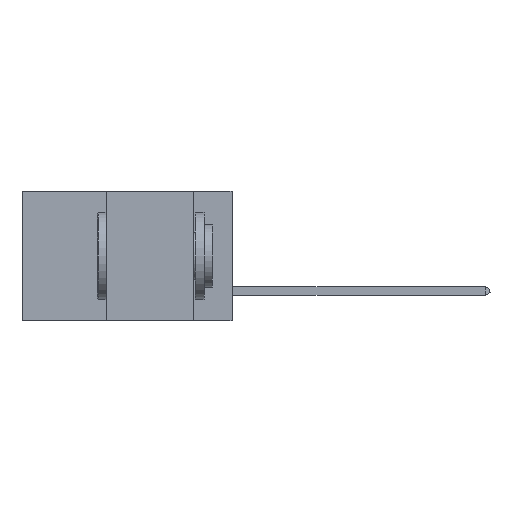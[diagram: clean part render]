
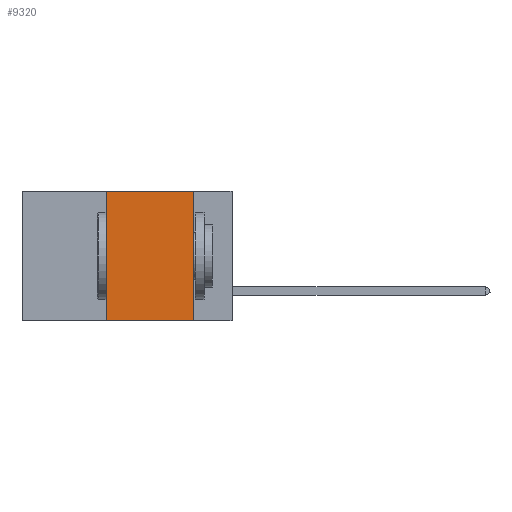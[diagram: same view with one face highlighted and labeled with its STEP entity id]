
A CAD part, left-side view. The second image highlights one B-rep face of the part: STEP entity #9320.
In plain terms, the highlighted planar face has unit normal (-1, 0, 0).
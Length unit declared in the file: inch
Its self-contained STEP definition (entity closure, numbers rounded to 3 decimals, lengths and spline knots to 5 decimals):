
#182 = VERTEX_POINT ( 'NONE', #21959 ) ;
#214 = EDGE_CURVE ( 'NONE', #22727, #182, #20677, .T. ) ;
#224 = PLANE ( 'NONE',  #19170 ) ;
#1705 = VECTOR ( 'NONE', #10304, 39.37008 ) ;
#1925 = VERTEX_POINT ( 'NONE', #24699 ) ;
#2066 = VECTOR ( 'NONE', #17421, 39.37008 ) ;
#2436 = CARTESIAN_POINT ( 'NONE',  ( 0., 0.36, 0. ) ) ;
#3633 = VERTEX_POINT ( 'NONE', #17122 ) ;
#4352 = EDGE_CURVE ( 'NONE', #1925, #22727, #13752, .T. ) ;
#5308 = EDGE_LOOP ( 'NONE', ( #23595, #17255, #15313, #19624 ) ) ;
#5347 = VECTOR ( 'NONE', #25000, 39.37008 ) ;
#5413 = CARTESIAN_POINT ( 'NONE',  ( 0., 0.6, -0.37 ) ) ;
#5674 = LINE ( 'NONE', #5413, #5347 ) ;
#6711 = CARTESIAN_POINT ( 'NONE',  ( 0., 0.6, 0. ) ) ;
#7829 = LINE ( 'NONE', #2436, #2066 ) ;
#8871 = DIRECTION ( 'NONE',  ( 0., 0., -1. ) ) ;
#9320 = ADVANCED_FACE ( 'NONE', ( #27726 ), #224, .F. ) ;
#10304 = DIRECTION ( 'NONE',  ( 0., 0., -1. ) ) ;
#13752 = LINE ( 'NONE', #24882, #23258 ) ;
#14034 = EDGE_CURVE ( 'NONE', #3633, #182, #5674, .T. ) ;
#15313 = ORIENTED_EDGE ( 'NONE', *, *, #24612, .F. ) ;
#17122 = CARTESIAN_POINT ( 'NONE',  ( 0., 0.36, -0.37 ) ) ;
#17255 = ORIENTED_EDGE ( 'NONE', *, *, #4352, .F. ) ;
#17421 = DIRECTION ( 'NONE',  ( 0., 0., 1. ) ) ;
#19170 = AXIS2_PLACEMENT_3D ( 'NONE', #6711, #20692, #8871 ) ;
#19624 = ORIENTED_EDGE ( 'NONE', *, *, #14034, .T. ) ;
#20264 = CARTESIAN_POINT ( 'NONE',  ( 0., 0.11, 0. ) ) ;
#20677 = LINE ( 'NONE', #20264, #1705 ) ;
#20692 = DIRECTION ( 'NONE',  ( 1., 0., 0. ) ) ;
#21959 = CARTESIAN_POINT ( 'NONE',  ( 0., 0.11, -0.37 ) ) ;
#21960 = CARTESIAN_POINT ( 'NONE',  ( 0., 0.11, 0. ) ) ;
#22699 = DIRECTION ( 'NONE',  ( 0., -1., 0. ) ) ;
#22727 = VERTEX_POINT ( 'NONE', #21960 ) ;
#23258 = VECTOR ( 'NONE', #22699, 39.37008 ) ;
#23595 = ORIENTED_EDGE ( 'NONE', *, *, #214, .F. ) ;
#24612 = EDGE_CURVE ( 'NONE', #3633, #1925, #7829, .T. ) ;
#24699 = CARTESIAN_POINT ( 'NONE',  ( 0., 0.36, 0. ) ) ;
#24882 = CARTESIAN_POINT ( 'NONE',  ( 0., 0.6, 0. ) ) ;
#25000 = DIRECTION ( 'NONE',  ( 0., -1., 0. ) ) ;
#27726 = FACE_OUTER_BOUND ( 'NONE', #5308, .T. ) ;
